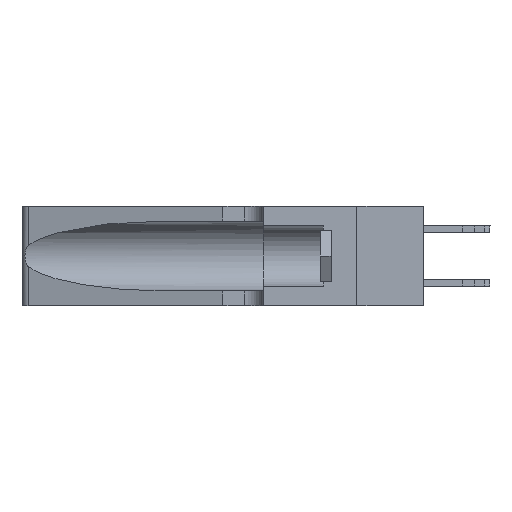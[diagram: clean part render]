
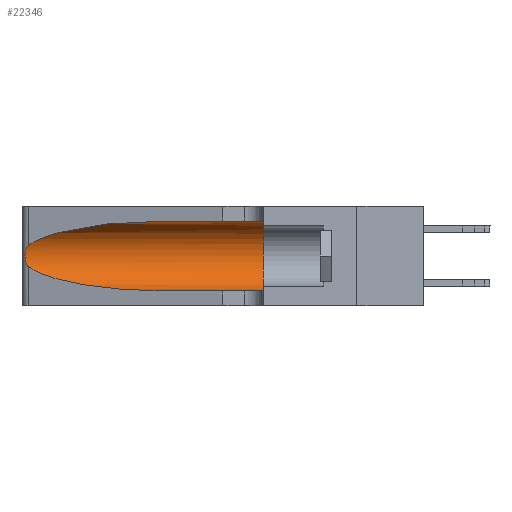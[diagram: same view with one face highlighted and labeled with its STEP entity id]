
A CAD part, left-side view. The second image highlights one B-rep face of the part: STEP entity #22346.
In plain terms, the highlighted cylindrical face has radius 3.308 mm (diameter 6.617 mm), a partial arc.
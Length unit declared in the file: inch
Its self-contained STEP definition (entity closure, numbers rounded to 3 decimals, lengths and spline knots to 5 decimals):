
#279 = CARTESIAN_POINT ( 'NONE',  ( 0.1305, 0.72297, 0.31525 ) ) ;
#707 = CARTESIAN_POINT ( 'NONE',  ( 0.25854, 1.2359, 0.20912 ) ) ;
#789 = CARTESIAN_POINT ( 'NONE',  ( 0.26075, 1.23896, 0.178 ) ) ;
#1297 = CARTESIAN_POINT ( 'NONE',  ( 0.18966, 0.96281, 0.05475 ) ) ;
#1324 = EDGE_CURVE ( 'NONE', #7998, #12852, #8264, .T. ) ;
#1779 = ORIENTED_EDGE ( 'NONE', *, *, #1324, .F. ) ;
#2942 = VERTEX_POINT ( 'NONE', #11703 ) ;
#3314 = CARTESIAN_POINT ( 'NONE',  ( 0.2373, 1.15595, 0.08982 ) ) ;
#4219 = B_SPLINE_CURVE_WITH_KNOTS ( 'NONE', 3,
 ( #11718, #4363, #6300, #6380, #707, #4612, #17318, #789, #11873, #19421, #15607, #17557, #17472, #9934 ),
 .UNSPECIFIED., .F., .F.,
 ( 4, 2, 2, 2, 2, 2, 4 ),
 ( 0., 0.00027, 0.00053, 0.00107, 0.0016, 0.00187, 0.00214 ),
 .UNSPECIFIED. ) ;
#4291 = VECTOR ( 'NONE', #22791, 39.37008 ) ;
#4363 = CARTESIAN_POINT ( 'NONE',  ( 0.25555, 1.22994, 0.2215 ) ) ;
#4612 = CARTESIAN_POINT ( 'NONE',  ( 0.26018, 1.23835, 0.19895 ) ) ;
#4954 = CARTESIAN_POINT ( 'NONE',  ( 0.1305, 0.35, 0.185 ) ) ;
#5552 =( BOUNDED_CURVE ( )  B_SPLINE_CURVE ( 3, ( #279, #7808, #6107, #9503 ),
 .UNSPECIFIED., .F., .F. ) 
 B_SPLINE_CURVE_WITH_KNOTS ( ( 4, 4 ),
 ( 1.5708, 2.84003 ),
 .UNSPECIFIED. ) 
 CURVE ( )  GEOMETRIC_REPRESENTATION_ITEM ( )  RATIONAL_B_SPLINE_CURVE ( ( 1., 0.87, 0.87, 1. ) ) 
 REPRESENTATION_ITEM ( '' )  );
#6107 = CARTESIAN_POINT ( 'NONE',  ( 0.2373, 1.15595, 0.28018 ) ) ;
#6300 = CARTESIAN_POINT ( 'NONE',  ( 0.25639, 1.23184, 0.21858 ) ) ;
#6380 = CARTESIAN_POINT ( 'NONE',  ( 0.25787, 1.23484, 0.2124 ) ) ;
#6444 = LINE ( 'NONE', #18312, #16872 ) ;
#7808 = CARTESIAN_POINT ( 'NONE',  ( 0.18966, 0.96281, 0.31525 ) ) ;
#7942 = EDGE_LOOP ( 'NONE', ( #17052, #19716, #16073, #17886, #1779, #12726 ) ) ;
#7998 = VERTEX_POINT ( 'NONE', #12164 ) ;
#8264 = CIRCLE ( 'NONE', #23986, 0.13025 ) ;
#9067 = DIRECTION ( 'NONE',  ( 0., -1., 0. ) ) ;
#9240 = CYLINDRICAL_SURFACE ( 'NONE', #15430, 0.13025 ) ;
#9503 = CARTESIAN_POINT ( 'NONE',  ( 0.25487, 1.22718, 0.22369 ) ) ;
#9844 =( BOUNDED_CURVE ( )  B_SPLINE_CURVE ( 3, ( #21629, #3314, #1297, #10742 ),
 .UNSPECIFIED., .F., .T. ) 
 B_SPLINE_CURVE_WITH_KNOTS ( ( 4, 4 ),
 ( 3.44316, 4.71239 ),
 .UNSPECIFIED. ) 
 CURVE ( )  GEOMETRIC_REPRESENTATION_ITEM ( )  RATIONAL_B_SPLINE_CURVE ( ( 1., 0.87, 0.87, 1. ) ) 
 REPRESENTATION_ITEM ( '' )  );
#9934 = CARTESIAN_POINT ( 'NONE',  ( 0.25487, 1.22718, 0.14631 ) ) ;
#10416 = DIRECTION ( 'NONE',  ( 0., -1., 0. ) ) ;
#10632 = EDGE_CURVE ( 'NONE', #14943, #11831, #9844, .T. ) ;
#10742 = CARTESIAN_POINT ( 'NONE',  ( 0.1305, 0.72297, 0.05475 ) ) ;
#11703 = CARTESIAN_POINT ( 'NONE',  ( 0.25487, 1.22718, 0.22369 ) ) ;
#11718 = CARTESIAN_POINT ( 'NONE',  ( 0.25487, 1.22718, 0.22369 ) ) ;
#11831 = VERTEX_POINT ( 'NONE', #15327 ) ;
#11873 = CARTESIAN_POINT ( 'NONE',  ( 0.26017, 1.23833, 0.17102 ) ) ;
#12164 = CARTESIAN_POINT ( 'NONE',  ( 0.1305, 0.35, 0.31525 ) ) ;
#12377 = DIRECTION ( 'NONE',  ( 0., 1., 0. ) ) ;
#12543 = DIRECTION ( 'NONE',  ( 0., 0., 1. ) ) ;
#12726 = ORIENTED_EDGE ( 'NONE', *, *, #22964, .F. ) ;
#12835 = CARTESIAN_POINT ( 'NONE',  ( 0.25487, 1.22718, 0.14631 ) ) ;
#12852 = VERTEX_POINT ( 'NONE', #22268 ) ;
#13244 = LINE ( 'NONE', #17437, #4291 ) ;
#13563 = FACE_OUTER_BOUND ( 'NONE', #7942, .T. ) ;
#13639 = EDGE_CURVE ( 'NONE', #21566, #2942, #5552, .T. ) ;
#14943 = VERTEX_POINT ( 'NONE', #12835 ) ;
#15327 = CARTESIAN_POINT ( 'NONE',  ( 0.1305, 0.72297, 0.05475 ) ) ;
#15430 = AXIS2_PLACEMENT_3D ( 'NONE', #17797, #10416, #21194 ) ;
#15607 = CARTESIAN_POINT ( 'NONE',  ( 0.25789, 1.23486, 0.15765 ) ) ;
#16073 = ORIENTED_EDGE ( 'NONE', *, *, #10632, .T. ) ;
#16872 = VECTOR ( 'NONE', #9067, 39.37008 ) ;
#17052 = ORIENTED_EDGE ( 'NONE', *, *, #13639, .T. ) ;
#17318 = CARTESIAN_POINT ( 'NONE',  ( 0.26075, 1.23896, 0.19203 ) ) ;
#17437 = CARTESIAN_POINT ( 'NONE',  ( 0.1305, 1.61858, 0.31525 ) ) ;
#17472 = CARTESIAN_POINT ( 'NONE',  ( 0.25555, 1.22993, 0.14849 ) ) ;
#17557 = CARTESIAN_POINT ( 'NONE',  ( 0.25639, 1.23186, 0.15144 ) ) ;
#17797 = CARTESIAN_POINT ( 'NONE',  ( 0.1305, 1.61858, 0.185 ) ) ;
#17886 = ORIENTED_EDGE ( 'NONE', *, *, #19587, .T. ) ;
#18312 = CARTESIAN_POINT ( 'NONE',  ( 0.1305, 1.61858, 0.05475 ) ) ;
#19421 = CARTESIAN_POINT ( 'NONE',  ( 0.25856, 1.23593, 0.16098 ) ) ;
#19587 = EDGE_CURVE ( 'NONE', #11831, #12852, #6444, .T. ) ;
#19716 = ORIENTED_EDGE ( 'NONE', *, *, #19796, .T. ) ;
#19796 = EDGE_CURVE ( 'NONE', #2942, #14943, #4219, .T. ) ;
#20984 = CARTESIAN_POINT ( 'NONE',  ( 0.1305, 0.72297, 0.31525 ) ) ;
#21194 = DIRECTION ( 'NONE',  ( 0., 0., -1. ) ) ;
#21566 = VERTEX_POINT ( 'NONE', #20984 ) ;
#21629 = CARTESIAN_POINT ( 'NONE',  ( 0.25487, 1.22718, 0.14631 ) ) ;
#22268 = CARTESIAN_POINT ( 'NONE',  ( 0.1305, 0.35, 0.05475 ) ) ;
#22346 = ADVANCED_FACE ( 'NONE', ( #13563 ), #9240, .F. ) ;
#22791 = DIRECTION ( 'NONE',  ( 0., -1., 0. ) ) ;
#22964 = EDGE_CURVE ( 'NONE', #21566, #7998, #13244, .T. ) ;
#23986 = AXIS2_PLACEMENT_3D ( 'NONE', #4954, #12377, #12543 ) ;
